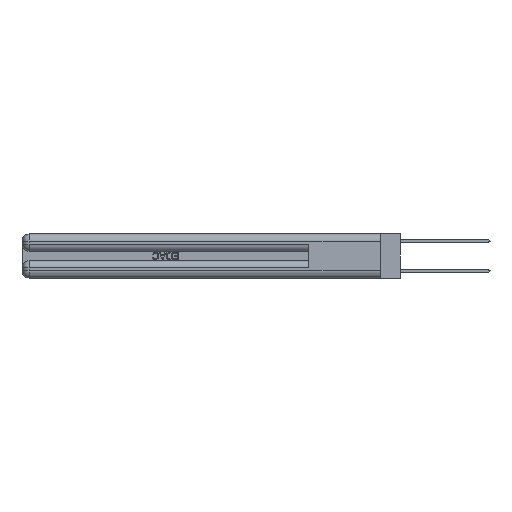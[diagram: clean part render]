
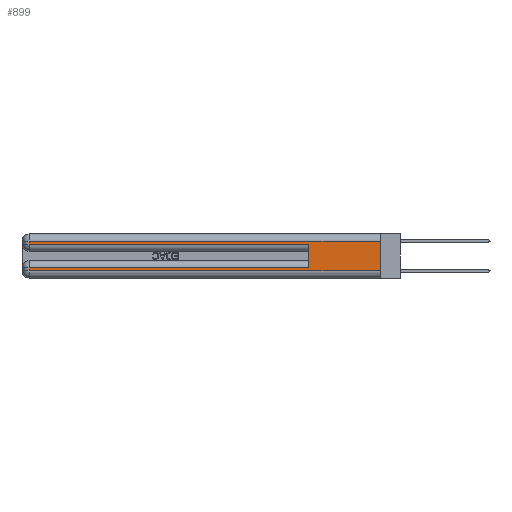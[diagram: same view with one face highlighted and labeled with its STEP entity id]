
A CAD part, left-side view. The second image highlights one B-rep face of the part: STEP entity #899.
In plain terms, the highlighted planar face has unit normal (-1, 0, 0).
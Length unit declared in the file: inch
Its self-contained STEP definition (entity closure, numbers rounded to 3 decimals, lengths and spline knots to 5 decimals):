
#472 = CARTESIAN_POINT ( 'NONE',  ( 0., 2.94, 0.085 ) ) ;
#565 = CARTESIAN_POINT ( 'NONE',  ( 0., 2.94, 0.37 ) ) ;
#899 = ADVANCED_FACE ( 'NONE', ( #12880 ), #7909, .F. ) ;
#1702 = VERTEX_POINT ( 'NONE', #472 ) ;
#2345 = VECTOR ( 'NONE', #28465, 39.37008 ) ;
#3722 = VECTOR ( 'NONE', #22499, 39.37008 ) ;
#3732 = EDGE_CURVE ( 'NONE', #10079, #29838, #22965, .T. ) ;
#4994 = DIRECTION ( 'NONE',  ( 0., 1., 0. ) ) ;
#5468 = LINE ( 'NONE', #565, #3722 ) ;
#5503 = CARTESIAN_POINT ( 'NONE',  ( 0., 2.94, 0.06 ) ) ;
#6623 = ORIENTED_EDGE ( 'NONE', *, *, #25306, .T. ) ;
#7287 = CARTESIAN_POINT ( 'NONE',  ( 0., 0., 0.085 ) ) ;
#7909 = PLANE ( 'NONE',  #30536 ) ;
#8500 = ORIENTED_EDGE ( 'NONE', *, *, #16901, .T. ) ;
#8686 = VERTEX_POINT ( 'NONE', #5503 ) ;
#9211 = VECTOR ( 'NONE', #10910, 39.37008 ) ;
#9253 = VECTOR ( 'NONE', #29242, 39.37008 ) ;
#9403 = VERTEX_POINT ( 'NONE', #24692 ) ;
#10079 = VERTEX_POINT ( 'NONE', #19772 ) ;
#10384 = EDGE_CURVE ( 'NONE', #8686, #31357, #14187, .T. ) ;
#10659 = CARTESIAN_POINT ( 'NONE',  ( 0., 0., 0.37 ) ) ;
#10910 = DIRECTION ( 'NONE',  ( 0., 0., -1. ) ) ;
#11854 = VECTOR ( 'NONE', #33607, 39.37008 ) ;
#12212 = CARTESIAN_POINT ( 'NONE',  ( 0., 0.6, 0.285 ) ) ;
#12880 = FACE_OUTER_BOUND ( 'NONE', #29197, .T. ) ;
#12970 = EDGE_CURVE ( 'NONE', #1702, #8686, #22516, .T. ) ;
#13162 = CARTESIAN_POINT ( 'NONE',  ( 0., 0., 0.31 ) ) ;
#13422 = DIRECTION ( 'NONE',  ( 0., 0., -1. ) ) ;
#14187 = LINE ( 'NONE', #15591, #15043 ) ;
#14980 = CARTESIAN_POINT ( 'NONE',  ( 0., 0., 0.06 ) ) ;
#15043 = VECTOR ( 'NONE', #18320, 39.37008 ) ;
#15232 = ORIENTED_EDGE ( 'NONE', *, *, #17915, .F. ) ;
#15349 = CARTESIAN_POINT ( 'NONE',  ( 0., 0.6, 0.085 ) ) ;
#15591 = CARTESIAN_POINT ( 'NONE',  ( 0., 0., 0.06 ) ) ;
#15977 = ORIENTED_EDGE ( 'NONE', *, *, #12970, .T. ) ;
#16242 = CARTESIAN_POINT ( 'NONE',  ( 0., 2.94, 0.31 ) ) ;
#16518 = LINE ( 'NONE', #7287, #9253 ) ;
#16901 = EDGE_CURVE ( 'NONE', #9403, #29548, #19116, .T. ) ;
#17327 = LINE ( 'NONE', #24503, #9211 ) ;
#17915 = EDGE_CURVE ( 'NONE', #10079, #31357, #17327, .T. ) ;
#18320 = DIRECTION ( 'NONE',  ( 0., -1., 0. ) ) ;
#19116 = LINE ( 'NONE', #28146, #11854 ) ;
#19772 = CARTESIAN_POINT ( 'NONE',  ( 0., 0., 0.31 ) ) ;
#20677 = EDGE_CURVE ( 'NONE', #27399, #1702, #16518, .T. ) ;
#20798 = VECTOR ( 'NONE', #29245, 39.37008 ) ;
#21019 = CARTESIAN_POINT ( 'NONE',  ( 0., 2.94, 0.37 ) ) ;
#22108 = VECTOR ( 'NONE', #4994, 39.37008 ) ;
#22499 = DIRECTION ( 'NONE',  ( 0., 0., -1. ) ) ;
#22516 = LINE ( 'NONE', #21019, #20798 ) ;
#22965 = LINE ( 'NONE', #13162, #22108 ) ;
#24191 = LINE ( 'NONE', #25707, #2345 ) ;
#24503 = CARTESIAN_POINT ( 'NONE',  ( 0., 0., 0.37 ) ) ;
#24692 = CARTESIAN_POINT ( 'NONE',  ( 0., 2.94, 0.285 ) ) ;
#24745 = ORIENTED_EDGE ( 'NONE', *, *, #3732, .T. ) ;
#25306 = EDGE_CURVE ( 'NONE', #29838, #9403, #5468, .T. ) ;
#25707 = CARTESIAN_POINT ( 'NONE',  ( 0., 0.6, 0.145 ) ) ;
#26231 = ORIENTED_EDGE ( 'NONE', *, *, #10384, .T. ) ;
#27270 = EDGE_CURVE ( 'NONE', #27399, #29548, #24191, .T. ) ;
#27399 = VERTEX_POINT ( 'NONE', #15349 ) ;
#28146 = CARTESIAN_POINT ( 'NONE',  ( 0., 0., 0.285 ) ) ;
#28465 = DIRECTION ( 'NONE',  ( 0., 0., 1. ) ) ;
#29197 = EDGE_LOOP ( 'NONE', ( #15232, #24745, #6623, #8500, #32444, #32882, #15977, #26231 ) ) ;
#29242 = DIRECTION ( 'NONE',  ( 0., 1., 0. ) ) ;
#29245 = DIRECTION ( 'NONE',  ( 0., 0., -1. ) ) ;
#29548 = VERTEX_POINT ( 'NONE', #12212 ) ;
#29721 = DIRECTION ( 'NONE',  ( 1., 0., 0. ) ) ;
#29838 = VERTEX_POINT ( 'NONE', #16242 ) ;
#30536 = AXIS2_PLACEMENT_3D ( 'NONE', #10659, #29721, #13422 ) ;
#31357 = VERTEX_POINT ( 'NONE', #14980 ) ;
#32444 = ORIENTED_EDGE ( 'NONE', *, *, #27270, .F. ) ;
#32882 = ORIENTED_EDGE ( 'NONE', *, *, #20677, .T. ) ;
#33607 = DIRECTION ( 'NONE',  ( 0., -1., 0. ) ) ;
